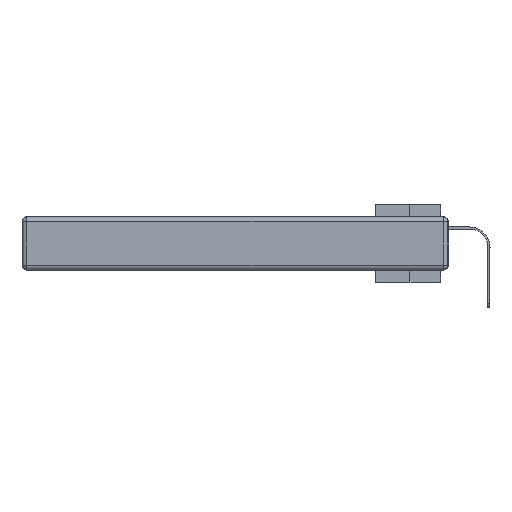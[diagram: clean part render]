
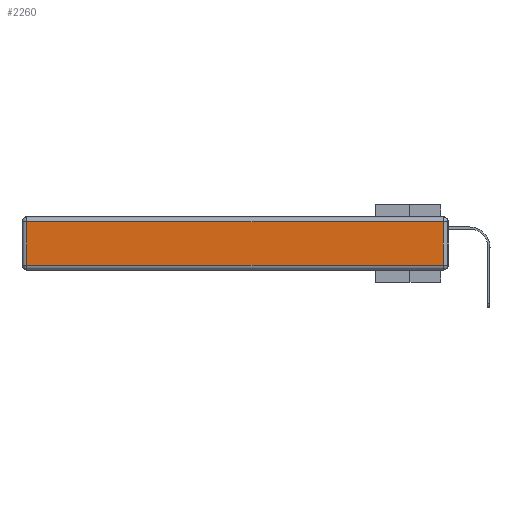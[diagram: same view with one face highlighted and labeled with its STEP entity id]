
A CAD part, left-side view. The second image highlights one B-rep face of the part: STEP entity #2260.
In plain terms, the highlighted planar face has unit normal (-1, 0, 0).
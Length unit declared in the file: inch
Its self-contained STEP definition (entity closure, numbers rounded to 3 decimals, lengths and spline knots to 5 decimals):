
#6 = VECTOR ( 'NONE', #11659, 39.37008 ) ;
#323 = ORIENTED_EDGE ( 'NONE', *, *, #29159, .T. ) ;
#547 = LINE ( 'NONE', #11557, #11970 ) ;
#647 = VERTEX_POINT ( 'NONE', #20748 ) ;
#2060 = EDGE_CURVE ( 'NONE', #8238, #26069, #3228, .T. ) ;
#2260 = ADVANCED_FACE ( 'NONE', ( #22408 ), #22260, .T. ) ;
#2353 = CARTESIAN_POINT ( 'NONE',  ( 0., 2.75, -0.03 ) ) ;
#2677 = CARTESIAN_POINT ( 'NONE',  ( 0., 2.72, -0.313 ) ) ;
#3228 = LINE ( 'NONE', #5218, #29797 ) ;
#3932 = LINE ( 'NONE', #8188, #8499 ) ;
#4385 = DIRECTION ( 'NONE',  ( 0., -1., 0. ) ) ;
#5218 = CARTESIAN_POINT ( 'NONE',  ( 0., 0.03, -0.343 ) ) ;
#5705 = ORIENTED_EDGE ( 'NONE', *, *, #11169, .T. ) ;
#6980 = AXIS2_PLACEMENT_3D ( 'NONE', #29261, #15407, #20119 ) ;
#8188 = CARTESIAN_POINT ( 'NONE',  ( 0., 2.72, -0.343 ) ) ;
#8238 = VERTEX_POINT ( 'NONE', #10888 ) ;
#8499 = VECTOR ( 'NONE', #19781, 39.37008 ) ;
#9196 = CARTESIAN_POINT ( 'NONE',  ( 0., 0.03, -0.03 ) ) ;
#10888 = CARTESIAN_POINT ( 'NONE',  ( 0., 0.03, -0.313 ) ) ;
#11169 = EDGE_CURVE ( 'NONE', #26069, #647, #28235, .T. ) ;
#11557 = CARTESIAN_POINT ( 'NONE',  ( 0., 0., -0.313 ) ) ;
#11659 = DIRECTION ( 'NONE',  ( 0., 1., 0. ) ) ;
#11970 = VECTOR ( 'NONE', #4385, 39.37008 ) ;
#15407 = DIRECTION ( 'NONE',  ( -1., 0., 0. ) ) ;
#15726 = VERTEX_POINT ( 'NONE', #2677 ) ;
#17277 = ORIENTED_EDGE ( 'NONE', *, *, #23942, .T. ) ;
#19521 = DIRECTION ( 'NONE',  ( 0., 0., 1. ) ) ;
#19781 = DIRECTION ( 'NONE',  ( 0., 0., -1. ) ) ;
#20119 = DIRECTION ( 'NONE',  ( 0., 0., 1. ) ) ;
#20748 = CARTESIAN_POINT ( 'NONE',  ( 0., 2.72, -0.03 ) ) ;
#22260 = PLANE ( 'NONE',  #6980 ) ;
#22408 = FACE_OUTER_BOUND ( 'NONE', #28656, .T. ) ;
#22875 = ORIENTED_EDGE ( 'NONE', *, *, #2060, .T. ) ;
#23942 = EDGE_CURVE ( 'NONE', #647, #15726, #3932, .T. ) ;
#26069 = VERTEX_POINT ( 'NONE', #9196 ) ;
#28235 = LINE ( 'NONE', #2353, #6 ) ;
#28656 = EDGE_LOOP ( 'NONE', ( #323, #22875, #5705, #17277 ) ) ;
#29159 = EDGE_CURVE ( 'NONE', #15726, #8238, #547, .T. ) ;
#29261 = CARTESIAN_POINT ( 'NONE',  ( 0., 0., -0.343 ) ) ;
#29797 = VECTOR ( 'NONE', #19521, 39.37008 ) ;
